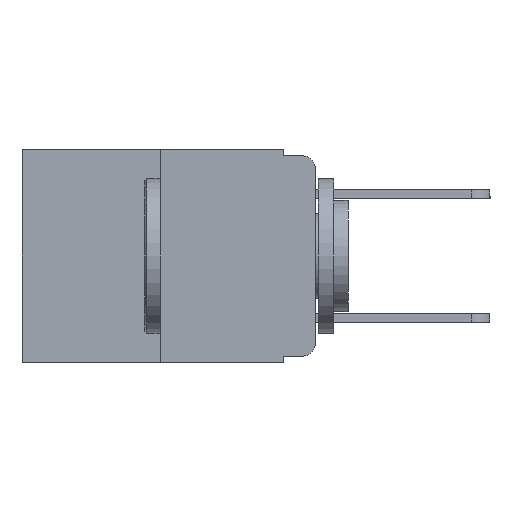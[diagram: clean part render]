
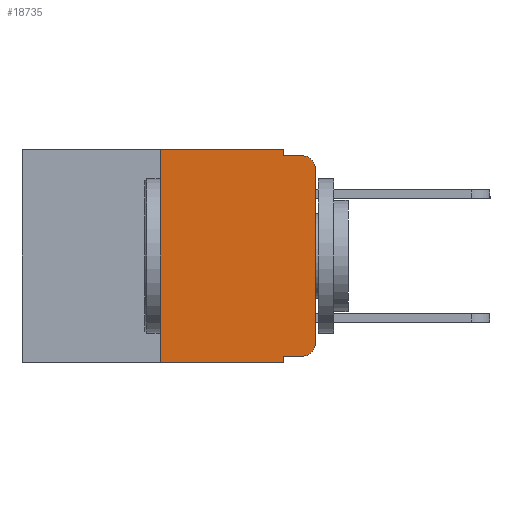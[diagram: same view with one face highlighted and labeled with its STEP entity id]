
A CAD part, left-side view. The second image highlights one B-rep face of the part: STEP entity #18735.
In plain terms, the highlighted planar face has unit normal (-1, 0, 0).
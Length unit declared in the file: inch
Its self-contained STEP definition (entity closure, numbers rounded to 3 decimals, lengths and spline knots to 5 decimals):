
#290 = LINE ( 'NONE', #9154, #16951 ) ;
#333 = AXIS2_PLACEMENT_3D ( 'NONE', #8577, #8513, #8321 ) ;
#768 = EDGE_CURVE ( 'NONE', #1636, #9081, #15646, .T. ) ;
#903 = DIRECTION ( 'NONE',  ( 0., -1., 0. ) ) ;
#946 = CIRCLE ( 'NONE', #333, 0.02 ) ;
#965 = CARTESIAN_POINT ( 'NONE',  ( 0., 0.02, -0.01 ) ) ;
#1349 = EDGE_CURVE ( 'NONE', #6185, #11639, #946, .T. ) ;
#1443 = LINE ( 'NONE', #14246, #9940 ) ;
#1636 = VERTEX_POINT ( 'NONE', #15021 ) ;
#1843 = VECTOR ( 'NONE', #9251, 39.37008 ) ;
#2145 = AXIS2_PLACEMENT_3D ( 'NONE', #13609, #2247, #13671 ) ;
#2247 = DIRECTION ( 'NONE',  ( 1., 0., 0. ) ) ;
#2337 = ORIENTED_EDGE ( 'NONE', *, *, #12428, .T. ) ;
#2373 = DIRECTION ( 'NONE',  ( 0., 0., 1. ) ) ;
#2384 = LINE ( 'NONE', #5825, #14771 ) ;
#2391 = DIRECTION ( 'NONE',  ( 0., -1., 0. ) ) ;
#3108 = ORIENTED_EDGE ( 'NONE', *, *, #1349, .T. ) ;
#3180 = VERTEX_POINT ( 'NONE', #4803 ) ;
#3839 = ORIENTED_EDGE ( 'NONE', *, *, #16547, .F. ) ;
#4803 = CARTESIAN_POINT ( 'NONE',  ( 0., 0.25, -0.343 ) ) ;
#5369 = ORIENTED_EDGE ( 'NONE', *, *, #17857, .F. ) ;
#5825 = CARTESIAN_POINT ( 'NONE',  ( 0., 0.051, -0.01 ) ) ;
#5881 = CARTESIAN_POINT ( 'NONE',  ( 0., 0.051, 0. ) ) ;
#6185 = VERTEX_POINT ( 'NONE', #15144 ) ;
#6215 = ORIENTED_EDGE ( 'NONE', *, *, #16572, .F. ) ;
#6288 = VECTOR ( 'NONE', #19046, 39.37008 ) ;
#6797 = LINE ( 'NONE', #17639, #6288 ) ;
#7326 = VERTEX_POINT ( 'NONE', #8877 ) ;
#8321 = DIRECTION ( 'NONE',  ( 0., 0., -1. ) ) ;
#8513 = DIRECTION ( 'NONE',  ( -1., 0., 0. ) ) ;
#8577 = CARTESIAN_POINT ( 'NONE',  ( 0., 0.02, -0.03 ) ) ;
#8877 = CARTESIAN_POINT ( 'NONE',  ( 0., 0.051, -0.01 ) ) ;
#9012 = VERTEX_POINT ( 'NONE', #16940 ) ;
#9030 = PLANE ( 'NONE',  #2145 ) ;
#9081 = VERTEX_POINT ( 'NONE', #9690 ) ;
#9154 = CARTESIAN_POINT ( 'NONE',  ( 0., 0.25, 0. ) ) ;
#9177 = DIRECTION ( 'NONE',  ( 0., -1., 0. ) ) ;
#9191 = ORIENTED_EDGE ( 'NONE', *, *, #10018, .F. ) ;
#9251 = DIRECTION ( 'NONE',  ( 0., -1., 0. ) ) ;
#9254 = CARTESIAN_POINT ( 'NONE',  ( 0., 0.473, -0.343 ) ) ;
#9513 = EDGE_CURVE ( 'NONE', #3180, #10423, #18743, .T. ) ;
#9690 = CARTESIAN_POINT ( 'NONE',  ( 0., 0., -0.313 ) ) ;
#9806 = VECTOR ( 'NONE', #903, 39.37008 ) ;
#9940 = VECTOR ( 'NONE', #15696, 39.37008 ) ;
#10018 = EDGE_CURVE ( 'NONE', #3180, #14165, #290, .T. ) ;
#10074 = LINE ( 'NONE', #5881, #14561 ) ;
#10423 = VERTEX_POINT ( 'NONE', #13873 ) ;
#10737 = ORIENTED_EDGE ( 'NONE', *, *, #9513, .T. ) ;
#11639 = VERTEX_POINT ( 'NONE', #965 ) ;
#11891 = VECTOR ( 'NONE', #9177, 39.37008 ) ;
#12428 = EDGE_CURVE ( 'NONE', #9081, #6185, #1443, .T. ) ;
#12513 = CARTESIAN_POINT ( 'NONE',  ( 0., 0.051, -0.333 ) ) ;
#13130 = VERTEX_POINT ( 'NONE', #17040 ) ;
#13334 = EDGE_LOOP ( 'NONE', ( #2337, #3108, #3839, #5369, #6215, #9191, #10737, #14069, #14877, #15576 ) ) ;
#13609 = CARTESIAN_POINT ( 'NONE',  ( 0., 0.473, 0. ) ) ;
#13671 = DIRECTION ( 'NONE',  ( 0., 0., -1. ) ) ;
#13790 = CARTESIAN_POINT ( 'NONE',  ( 0., 0.473, 0. ) ) ;
#13836 = DIRECTION ( 'NONE',  ( 0., 0., -1. ) ) ;
#13843 = LINE ( 'NONE', #12513, #9806 ) ;
#13873 = CARTESIAN_POINT ( 'NONE',  ( 0., 0.051, -0.343 ) ) ;
#14069 = ORIENTED_EDGE ( 'NONE', *, *, #15166, .F. ) ;
#14165 = VERTEX_POINT ( 'NONE', #15836 ) ;
#14246 = CARTESIAN_POINT ( 'NONE',  ( 0., 0., 0. ) ) ;
#14561 = VECTOR ( 'NONE', #13836, 39.37008 ) ;
#14771 = VECTOR ( 'NONE', #2391, 39.37008 ) ;
#14877 = ORIENTED_EDGE ( 'NONE', *, *, #19558, .T. ) ;
#15021 = CARTESIAN_POINT ( 'NONE',  ( 0., 0.02, -0.333 ) ) ;
#15144 = CARTESIAN_POINT ( 'NONE',  ( 0., 0., -0.03 ) ) ;
#15166 = EDGE_CURVE ( 'NONE', #9012, #10423, #10074, .T. ) ;
#15220 = LINE ( 'NONE', #13790, #1843 ) ;
#15576 = ORIENTED_EDGE ( 'NONE', *, *, #768, .T. ) ;
#15646 = CIRCLE ( 'NONE', #17074, 0.02 ) ;
#15696 = DIRECTION ( 'NONE',  ( 0., 0., 1. ) ) ;
#15836 = CARTESIAN_POINT ( 'NONE',  ( 0., 0.25, 0. ) ) ;
#16547 = EDGE_CURVE ( 'NONE', #7326, #11639, #2384, .T. ) ;
#16572 = EDGE_CURVE ( 'NONE', #14165, #13130, #15220, .T. ) ;
#16692 = DIRECTION ( 'NONE',  ( 0., 0., -1. ) ) ;
#16791 = DIRECTION ( 'NONE',  ( -1., 0., 0. ) ) ;
#16940 = CARTESIAN_POINT ( 'NONE',  ( 0., 0.051, -0.333 ) ) ;
#16951 = VECTOR ( 'NONE', #2373, 39.37008 ) ;
#17040 = CARTESIAN_POINT ( 'NONE',  ( 0., 0.051, 0. ) ) ;
#17074 = AXIS2_PLACEMENT_3D ( 'NONE', #19051, #16791, #16692 ) ;
#17639 = CARTESIAN_POINT ( 'NONE',  ( 0., 0.051, 0. ) ) ;
#17857 = EDGE_CURVE ( 'NONE', #13130, #7326, #6797, .T. ) ;
#18735 = ADVANCED_FACE ( 'NONE', ( #19249 ), #9030, .F. ) ;
#18743 = LINE ( 'NONE', #9254, #11891 ) ;
#19046 = DIRECTION ( 'NONE',  ( 0., 0., -1. ) ) ;
#19051 = CARTESIAN_POINT ( 'NONE',  ( 0., 0.02, -0.313 ) ) ;
#19249 = FACE_OUTER_BOUND ( 'NONE', #13334, .T. ) ;
#19558 = EDGE_CURVE ( 'NONE', #9012, #1636, #13843, .T. ) ;
